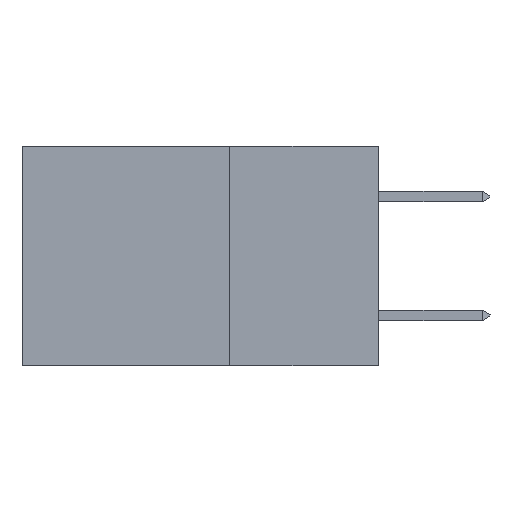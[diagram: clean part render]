
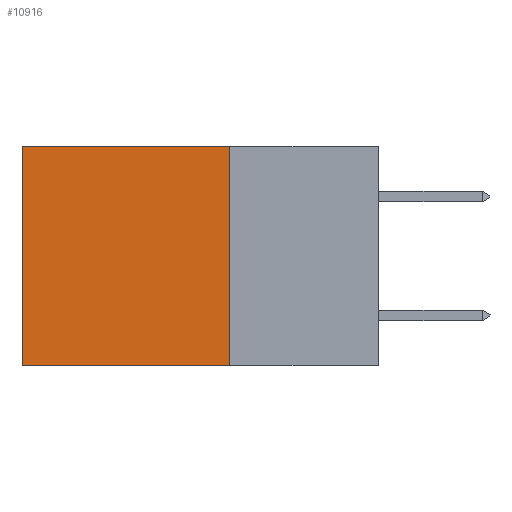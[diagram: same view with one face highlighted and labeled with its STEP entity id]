
A CAD part, left-side view. The second image highlights one B-rep face of the part: STEP entity #10916.
In plain terms, the highlighted planar face has unit normal (-1, 0, 0).
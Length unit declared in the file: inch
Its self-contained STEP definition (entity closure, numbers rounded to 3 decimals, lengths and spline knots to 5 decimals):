
#76 = DIRECTION ( 'NONE',  ( 0., 1., 0. ) ) ;
#104 = ORIENTED_EDGE ( 'NONE', *, *, #8069, .F. ) ;
#221 = EDGE_CURVE ( 'NONE', #15156, #11713, #7462, .T. ) ;
#592 = ORIENTED_EDGE ( 'NONE', *, *, #926, .F. ) ;
#926 = EDGE_CURVE ( 'NONE', #15156, #3637, #1158, .T. ) ;
#1158 = LINE ( 'NONE', #4578, #15987 ) ;
#1290 = AXIS2_PLACEMENT_3D ( 'NONE', #10934, #13957, #7941 ) ;
#1302 = DIRECTION ( 'NONE',  ( 0., 1., 0. ) ) ;
#1953 = VERTEX_POINT ( 'NONE', #7077 ) ;
#2019 = CARTESIAN_POINT ( 'NONE',  ( 0.298, 0.25, 0. ) ) ;
#2990 = CARTESIAN_POINT ( 'NONE',  ( 0.298, 0.25, -0.37 ) ) ;
#3637 = VERTEX_POINT ( 'NONE', #14858 ) ;
#3800 = LINE ( 'NONE', #2990, #10088 ) ;
#4578 = CARTESIAN_POINT ( 'NONE',  ( 0.298, 0.25, 0. ) ) ;
#5515 = CARTESIAN_POINT ( 'NONE',  ( 0.298, 0.6, 0. ) ) ;
#6453 = PLANE ( 'NONE',  #1290 ) ;
#7077 = CARTESIAN_POINT ( 'NONE',  ( 0.298, 0.6, -0.37 ) ) ;
#7204 = FACE_OUTER_BOUND ( 'NONE', #8411, .T. ) ;
#7462 = LINE ( 'NONE', #17315, #12799 ) ;
#7602 = CARTESIAN_POINT ( 'NONE',  ( 0.298, 0.6, 0. ) ) ;
#7941 = DIRECTION ( 'NONE',  ( 0., 0., -1. ) ) ;
#7965 = VECTOR ( 'NONE', #10245, 39.37008 ) ;
#8069 = EDGE_CURVE ( 'NONE', #3637, #1953, #3800, .T. ) ;
#8411 = EDGE_LOOP ( 'NONE', ( #11016, #104, #592, #9422 ) ) ;
#9422 = ORIENTED_EDGE ( 'NONE', *, *, #221, .T. ) ;
#10088 = VECTOR ( 'NONE', #76, 39.37008 ) ;
#10245 = DIRECTION ( 'NONE',  ( 0., 0., -1. ) ) ;
#10916 = ADVANCED_FACE ( 'NONE', ( #7204 ), #6453, .F. ) ;
#10934 = CARTESIAN_POINT ( 'NONE',  ( 0.298, 0.25, 0. ) ) ;
#11016 = ORIENTED_EDGE ( 'NONE', *, *, #18766, .T. ) ;
#11713 = VERTEX_POINT ( 'NONE', #7602 ) ;
#12799 = VECTOR ( 'NONE', #1302, 39.37008 ) ;
#13957 = DIRECTION ( 'NONE',  ( 1., 0., 0. ) ) ;
#14858 = CARTESIAN_POINT ( 'NONE',  ( 0.298, 0.25, -0.37 ) ) ;
#15156 = VERTEX_POINT ( 'NONE', #2019 ) ;
#15987 = VECTOR ( 'NONE', #17860, 39.37008 ) ;
#17315 = CARTESIAN_POINT ( 'NONE',  ( 0.298, 0.25, 0. ) ) ;
#17418 = LINE ( 'NONE', #5515, #7965 ) ;
#17860 = DIRECTION ( 'NONE',  ( 0., 0., -1. ) ) ;
#18766 = EDGE_CURVE ( 'NONE', #11713, #1953, #17418, .T. ) ;
